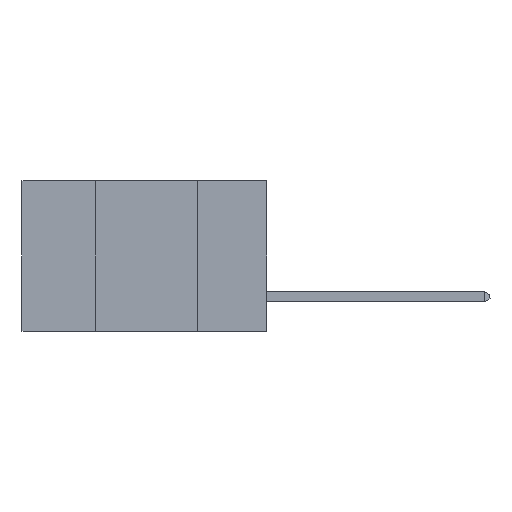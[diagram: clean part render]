
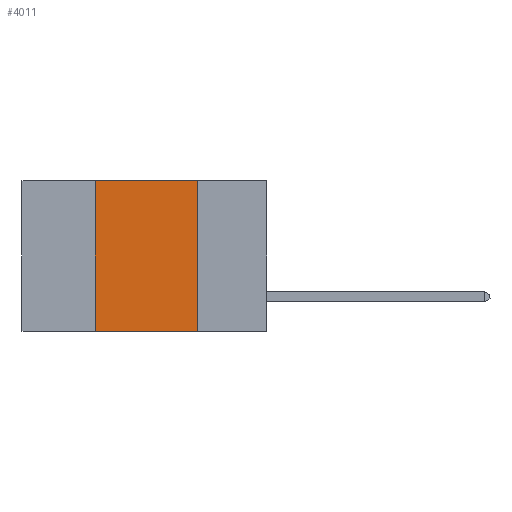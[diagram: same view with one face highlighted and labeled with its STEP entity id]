
A CAD part, left-side view. The second image highlights one B-rep face of the part: STEP entity #4011.
In plain terms, the highlighted planar face has unit normal (-1, 0, 0).
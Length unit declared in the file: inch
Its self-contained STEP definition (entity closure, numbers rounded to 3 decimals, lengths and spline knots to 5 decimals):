
#246 = ORIENTED_EDGE ( 'NONE', *, *, #5793, .F. ) ;
#291 = CARTESIAN_POINT ( 'NONE',  ( 0., 0.17, -0.37 ) ) ;
#547 = VERTEX_POINT ( 'NONE', #291 ) ;
#844 = CARTESIAN_POINT ( 'NONE',  ( 0., 0.42, 0. ) ) ;
#1189 = VECTOR ( 'NONE', #3110, 39.37008 ) ;
#1414 = VERTEX_POINT ( 'NONE', #2178 ) ;
#1440 = CARTESIAN_POINT ( 'NONE',  ( 0., 0.17, 0. ) ) ;
#1483 = DIRECTION ( 'NONE',  ( 0., 0., 1. ) ) ;
#1987 = VECTOR ( 'NONE', #1483, 39.37008 ) ;
#2178 = CARTESIAN_POINT ( 'NONE',  ( 0., 0.42, -0.37 ) ) ;
#2324 = CARTESIAN_POINT ( 'NONE',  ( 0., 0.42, 0. ) ) ;
#2355 = CARTESIAN_POINT ( 'NONE',  ( 0., 0.6, 0. ) ) ;
#2472 = VERTEX_POINT ( 'NONE', #4321 ) ;
#2480 = ORIENTED_EDGE ( 'NONE', *, *, #3930, .F. ) ;
#3110 = DIRECTION ( 'NONE',  ( 0., 0., -1. ) ) ;
#3706 = ORIENTED_EDGE ( 'NONE', *, *, #7717, .F. ) ;
#3864 = DIRECTION ( 'NONE',  ( 0., -1., 0. ) ) ;
#3900 = LINE ( 'NONE', #1440, #1189 ) ;
#3930 = EDGE_CURVE ( 'NONE', #2472, #547, #3900, .T. ) ;
#3975 = PLANE ( 'NONE',  #6084 ) ;
#4011 = ADVANCED_FACE ( 'NONE', ( #6835 ), #3975, .F. ) ;
#4321 = CARTESIAN_POINT ( 'NONE',  ( 0., 0.17, 0. ) ) ;
#4463 = LINE ( 'NONE', #5930, #6093 ) ;
#4767 = DIRECTION ( 'NONE',  ( 0., 0., -1. ) ) ;
#5719 = LINE ( 'NONE', #7710, #7480 ) ;
#5793 = EDGE_CURVE ( 'NONE', #1414, #8741, #8081, .T. ) ;
#5930 = CARTESIAN_POINT ( 'NONE',  ( 0., 0.6, 0. ) ) ;
#6084 = AXIS2_PLACEMENT_3D ( 'NONE', #2355, #9261, #4767 ) ;
#6093 = VECTOR ( 'NONE', #9568, 39.37008 ) ;
#6835 = FACE_OUTER_BOUND ( 'NONE', #7734, .T. ) ;
#7480 = VECTOR ( 'NONE', #3864, 39.37008 ) ;
#7710 = CARTESIAN_POINT ( 'NONE',  ( 0., 0.6, -0.37 ) ) ;
#7717 = EDGE_CURVE ( 'NONE', #8741, #2472, #4463, .T. ) ;
#7734 = EDGE_LOOP ( 'NONE', ( #2480, #3706, #246, #8020 ) ) ;
#7978 = EDGE_CURVE ( 'NONE', #1414, #547, #5719, .T. ) ;
#8020 = ORIENTED_EDGE ( 'NONE', *, *, #7978, .T. ) ;
#8081 = LINE ( 'NONE', #2324, #1987 ) ;
#8741 = VERTEX_POINT ( 'NONE', #844 ) ;
#9261 = DIRECTION ( 'NONE',  ( 1., 0., 0. ) ) ;
#9568 = DIRECTION ( 'NONE',  ( 0., -1., 0. ) ) ;
